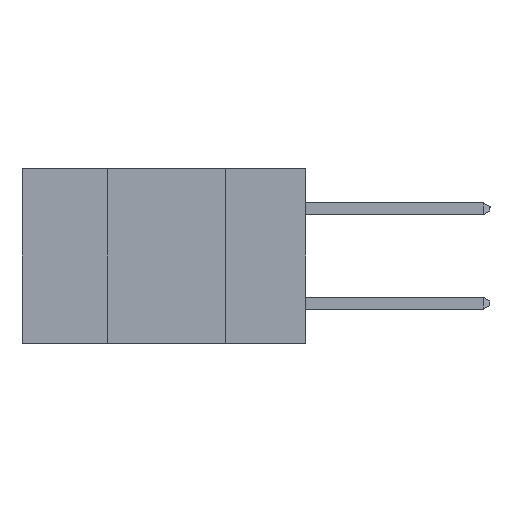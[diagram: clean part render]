
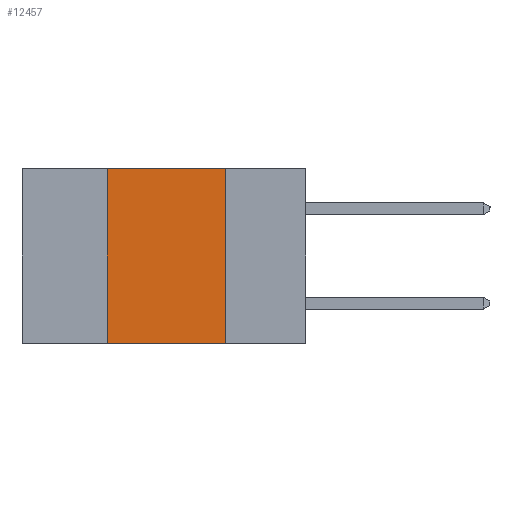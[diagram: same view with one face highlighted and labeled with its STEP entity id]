
A CAD part, left-side view. The second image highlights one B-rep face of the part: STEP entity #12457.
In plain terms, the highlighted planar face has unit normal (-1, 0, 0).
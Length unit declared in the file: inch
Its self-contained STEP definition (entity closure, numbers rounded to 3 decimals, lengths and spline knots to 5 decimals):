
#104 = CARTESIAN_POINT ( 'NONE',  ( 0., 0.17, -0.37 ) ) ;
#426 = ORIENTED_EDGE ( 'NONE', *, *, #11639, .F. ) ;
#435 = CARTESIAN_POINT ( 'NONE',  ( 0., 0.42, 0. ) ) ;
#1299 = VERTEX_POINT ( 'NONE', #26181 ) ;
#1435 = PLANE ( 'NONE',  #4389 ) ;
#4389 = AXIS2_PLACEMENT_3D ( 'NONE', #21563, #19807, #17509 ) ;
#4722 = ORIENTED_EDGE ( 'NONE', *, *, #21862, .T. ) ;
#4879 = VECTOR ( 'NONE', #21528, 39.37008 ) ;
#5165 = DIRECTION ( 'NONE',  ( 0., 0., 1. ) ) ;
#6701 = EDGE_LOOP ( 'NONE', ( #426, #12129, #19959, #4722 ) ) ;
#7175 = CARTESIAN_POINT ( 'NONE',  ( 0., 0.42, -0.37 ) ) ;
#8094 = LINE ( 'NONE', #20286, #12550 ) ;
#11639 = EDGE_CURVE ( 'NONE', #12856, #21863, #8094, .T. ) ;
#12024 = LINE ( 'NONE', #24849, #14514 ) ;
#12129 = ORIENTED_EDGE ( 'NONE', *, *, #16239, .F. ) ;
#12159 = DIRECTION ( 'NONE',  ( 0., 0., -1. ) ) ;
#12457 = ADVANCED_FACE ( 'NONE', ( #19946 ), #1435, .F. ) ;
#12550 = VECTOR ( 'NONE', #12159, 39.37008 ) ;
#12856 = VERTEX_POINT ( 'NONE', #23294 ) ;
#14514 = VECTOR ( 'NONE', #24717, 39.37008 ) ;
#16239 = EDGE_CURVE ( 'NONE', #24150, #12856, #17322, .T. ) ;
#17322 = LINE ( 'NONE', #23563, #4879 ) ;
#17509 = DIRECTION ( 'NONE',  ( 0., 0., -1. ) ) ;
#18140 = LINE ( 'NONE', #7175, #26178 ) ;
#19807 = DIRECTION ( 'NONE',  ( 1., 0., 0. ) ) ;
#19946 = FACE_OUTER_BOUND ( 'NONE', #6701, .T. ) ;
#19959 = ORIENTED_EDGE ( 'NONE', *, *, #21210, .F. ) ;
#20286 = CARTESIAN_POINT ( 'NONE',  ( 0., 0.17, -0.37 ) ) ;
#21210 = EDGE_CURVE ( 'NONE', #1299, #24150, #18140, .T. ) ;
#21528 = DIRECTION ( 'NONE',  ( 0., -1., 0. ) ) ;
#21563 = CARTESIAN_POINT ( 'NONE',  ( 0., 0.6, 0. ) ) ;
#21862 = EDGE_CURVE ( 'NONE', #1299, #21863, #12024, .T. ) ;
#21863 = VERTEX_POINT ( 'NONE', #104 ) ;
#23294 = CARTESIAN_POINT ( 'NONE',  ( 0., 0.17, 0. ) ) ;
#23563 = CARTESIAN_POINT ( 'NONE',  ( 0., 0.6, 0. ) ) ;
#24150 = VERTEX_POINT ( 'NONE', #435 ) ;
#24717 = DIRECTION ( 'NONE',  ( 0., -1., 0. ) ) ;
#24849 = CARTESIAN_POINT ( 'NONE',  ( 0., 0.6, -0.37 ) ) ;
#26178 = VECTOR ( 'NONE', #5165, 39.37008 ) ;
#26181 = CARTESIAN_POINT ( 'NONE',  ( 0., 0.42, -0.37 ) ) ;
